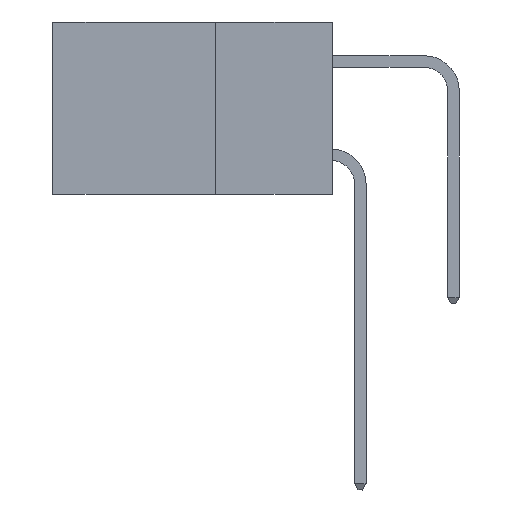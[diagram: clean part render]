
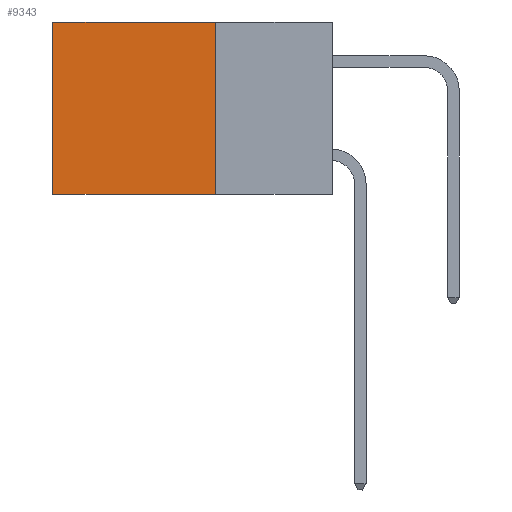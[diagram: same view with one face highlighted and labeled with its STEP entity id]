
A CAD part, left-side view. The second image highlights one B-rep face of the part: STEP entity #9343.
In plain terms, the highlighted planar face has unit normal (-1, 0, 0).
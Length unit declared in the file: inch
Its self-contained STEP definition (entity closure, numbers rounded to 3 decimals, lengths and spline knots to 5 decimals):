
#630 = CARTESIAN_POINT ( 'NONE',  ( 0.298, 0.25, -0.37 ) ) ;
#1307 = LINE ( 'NONE', #25561, #12514 ) ;
#2755 = CARTESIAN_POINT ( 'NONE',  ( 0.298, 0.25, 0. ) ) ;
#2807 = VERTEX_POINT ( 'NONE', #24988 ) ;
#3201 = AXIS2_PLACEMENT_3D ( 'NONE', #2755, #17482, #4870 ) ;
#4055 = CARTESIAN_POINT ( 'NONE',  ( 0.298, 0.25, 0. ) ) ;
#4147 = EDGE_CURVE ( 'NONE', #17389, #22954, #6279, .T. ) ;
#4870 = DIRECTION ( 'NONE',  ( 0., 0., -1. ) ) ;
#6279 = LINE ( 'NONE', #27145, #26577 ) ;
#9003 = CARTESIAN_POINT ( 'NONE',  ( 0.298, 0.6, 0. ) ) ;
#9067 = VECTOR ( 'NONE', #18871, 39.37008 ) ;
#9343 = ADVANCED_FACE ( 'NONE', ( #10639 ), #25752, .F. ) ;
#9645 = VERTEX_POINT ( 'NONE', #20443 ) ;
#10639 = FACE_OUTER_BOUND ( 'NONE', #17817, .T. ) ;
#11304 = ORIENTED_EDGE ( 'NONE', *, *, #21989, .F. ) ;
#12514 = VECTOR ( 'NONE', #13108, 39.37008 ) ;
#13108 = DIRECTION ( 'NONE',  ( 0., 1., 0. ) ) ;
#14191 = LINE ( 'NONE', #9003, #23942 ) ;
#14453 = ORIENTED_EDGE ( 'NONE', *, *, #4147, .F. ) ;
#14624 = LINE ( 'NONE', #16774, #9067 ) ;
#15338 = DIRECTION ( 'NONE',  ( 0., 0., -1. ) ) ;
#16774 = CARTESIAN_POINT ( 'NONE',  ( 0.298, 0.25, 0. ) ) ;
#17389 = VERTEX_POINT ( 'NONE', #4055 ) ;
#17420 = EDGE_CURVE ( 'NONE', #17389, #9645, #14624, .T. ) ;
#17482 = DIRECTION ( 'NONE',  ( 1., 0., 0. ) ) ;
#17817 = EDGE_LOOP ( 'NONE', ( #18908, #11304, #14453, #22604 ) ) ;
#18870 = DIRECTION ( 'NONE',  ( 0., 0., -1. ) ) ;
#18871 = DIRECTION ( 'NONE',  ( 0., 1., 0. ) ) ;
#18908 = ORIENTED_EDGE ( 'NONE', *, *, #21382, .T. ) ;
#20443 = CARTESIAN_POINT ( 'NONE',  ( 0.298, 0.6, 0. ) ) ;
#21382 = EDGE_CURVE ( 'NONE', #9645, #2807, #14191, .T. ) ;
#21989 = EDGE_CURVE ( 'NONE', #22954, #2807, #1307, .T. ) ;
#22604 = ORIENTED_EDGE ( 'NONE', *, *, #17420, .T. ) ;
#22954 = VERTEX_POINT ( 'NONE', #630 ) ;
#23942 = VECTOR ( 'NONE', #15338, 39.37008 ) ;
#24988 = CARTESIAN_POINT ( 'NONE',  ( 0.298, 0.6, -0.37 ) ) ;
#25561 = CARTESIAN_POINT ( 'NONE',  ( 0.298, 0.25, -0.37 ) ) ;
#25752 = PLANE ( 'NONE',  #3201 ) ;
#26577 = VECTOR ( 'NONE', #18870, 39.37008 ) ;
#27145 = CARTESIAN_POINT ( 'NONE',  ( 0.298, 0.25, 0. ) ) ;
